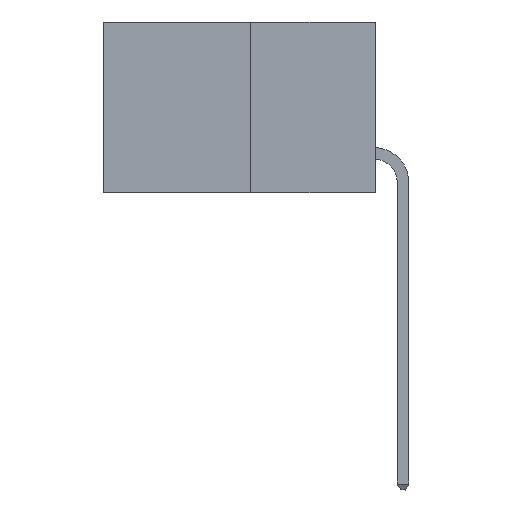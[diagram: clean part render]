
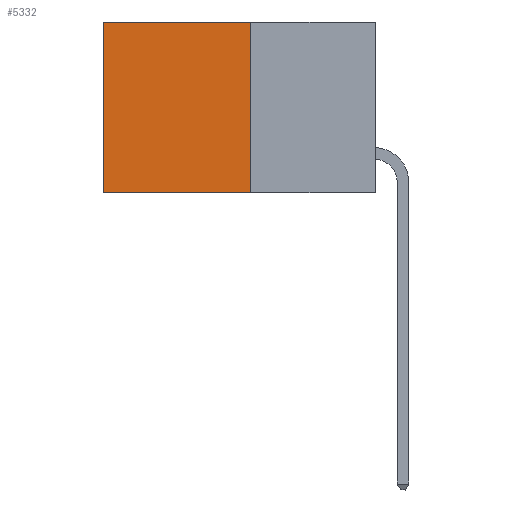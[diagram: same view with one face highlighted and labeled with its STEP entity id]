
A CAD part, left-side view. The second image highlights one B-rep face of the part: STEP entity #5332.
In plain terms, the highlighted planar face has unit normal (-1, 0, 0).
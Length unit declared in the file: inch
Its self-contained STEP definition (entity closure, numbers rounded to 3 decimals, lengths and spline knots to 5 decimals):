
#94 = DIRECTION ( 'NONE',  ( 0., 1., 0. ) ) ;
#341 = EDGE_CURVE ( 'NONE', #3410, #2104, #5234, .T. ) ;
#565 = DIRECTION ( 'NONE',  ( 1., 0., 0. ) ) ;
#782 = CARTESIAN_POINT ( 'NONE',  ( 0.277, 0.27, -0.37 ) ) ;
#974 = CARTESIAN_POINT ( 'NONE',  ( 0.277, 0.27, -0.37 ) ) ;
#1093 = EDGE_CURVE ( 'NONE', #6370, #7621, #7099, .T. ) ;
#1882 = EDGE_CURVE ( 'NONE', #7621, #2104, #2993, .T. ) ;
#2104 = VERTEX_POINT ( 'NONE', #6328 ) ;
#2703 = ORIENTED_EDGE ( 'NONE', *, *, #1882, .F. ) ;
#2977 = CARTESIAN_POINT ( 'NONE',  ( 0.277, 0.59, 0. ) ) ;
#2993 = LINE ( 'NONE', #782, #4306 ) ;
#3172 = AXIS2_PLACEMENT_3D ( 'NONE', #5702, #565, #4121 ) ;
#3364 = VECTOR ( 'NONE', #4819, 39.37008 ) ;
#3393 = ORIENTED_EDGE ( 'NONE', *, *, #1093, .F. ) ;
#3410 = VERTEX_POINT ( 'NONE', #2977 ) ;
#3715 = DIRECTION ( 'NONE',  ( 0., 0., -1. ) ) ;
#4121 = DIRECTION ( 'NONE',  ( 0., 0., -1. ) ) ;
#4306 = VECTOR ( 'NONE', #94, 39.37008 ) ;
#4411 = ORIENTED_EDGE ( 'NONE', *, *, #341, .T. ) ;
#4819 = DIRECTION ( 'NONE',  ( 0., 0., -1. ) ) ;
#5095 = PLANE ( 'NONE',  #3172 ) ;
#5234 = LINE ( 'NONE', #6730, #3364 ) ;
#5332 = ADVANCED_FACE ( 'NONE', ( #5903 ), #5095, .F. ) ;
#5599 = EDGE_CURVE ( 'NONE', #6370, #3410, #7071, .T. ) ;
#5648 = ORIENTED_EDGE ( 'NONE', *, *, #5599, .T. ) ;
#5664 = CARTESIAN_POINT ( 'NONE',  ( 0.277, 0.27, -0.37 ) ) ;
#5682 = VECTOR ( 'NONE', #3715, 39.37008 ) ;
#5702 = CARTESIAN_POINT ( 'NONE',  ( 0.277, 0.27, -0.37 ) ) ;
#5903 = FACE_OUTER_BOUND ( 'NONE', #7088, .T. ) ;
#6328 = CARTESIAN_POINT ( 'NONE',  ( 0.277, 0.59, -0.37 ) ) ;
#6370 = VERTEX_POINT ( 'NONE', #7413 ) ;
#6553 = CARTESIAN_POINT ( 'NONE',  ( 0.277, 0.27, 0. ) ) ;
#6730 = CARTESIAN_POINT ( 'NONE',  ( 0.277, 0.59, -0.37 ) ) ;
#6911 = VECTOR ( 'NONE', #7261, 39.37008 ) ;
#7071 = LINE ( 'NONE', #6553, #6911 ) ;
#7088 = EDGE_LOOP ( 'NONE', ( #4411, #2703, #3393, #5648 ) ) ;
#7099 = LINE ( 'NONE', #974, #5682 ) ;
#7261 = DIRECTION ( 'NONE',  ( 0., 1., 0. ) ) ;
#7413 = CARTESIAN_POINT ( 'NONE',  ( 0.277, 0.27, 0. ) ) ;
#7621 = VERTEX_POINT ( 'NONE', #5664 ) ;
